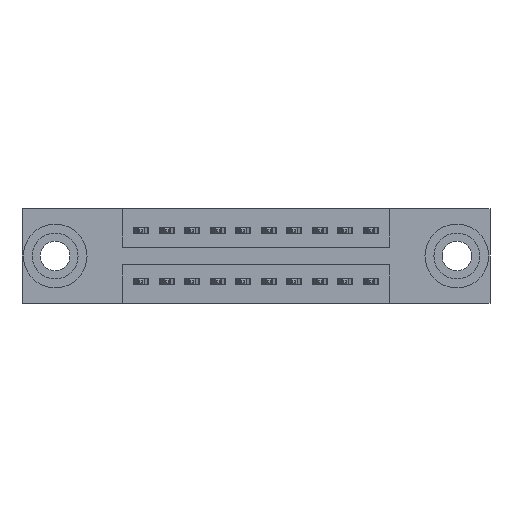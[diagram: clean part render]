
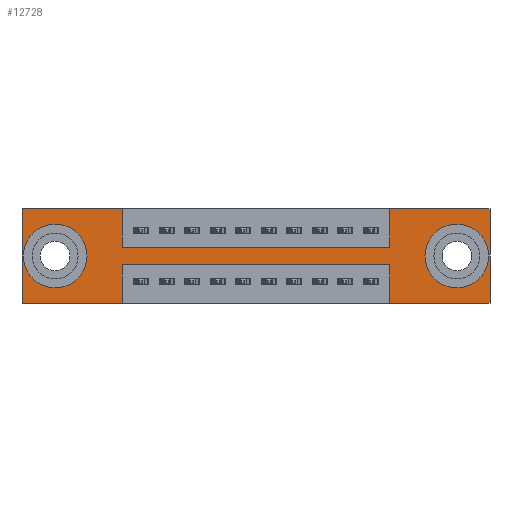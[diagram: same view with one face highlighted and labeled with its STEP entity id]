
A CAD part, front view. The second image highlights one B-rep face of the part: STEP entity #12728.
In plain terms, the highlighted planar face has unit normal (0, -1, 0).
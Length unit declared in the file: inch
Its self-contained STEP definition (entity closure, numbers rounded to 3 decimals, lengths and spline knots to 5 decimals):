
#14 = AXIS2_PLACEMENT_3D ( 'NONE', #4909, #11758, #6761 ) ;
#334 = CARTESIAN_POINT ( 'NONE',  ( 0.13, 0., -0.263 ) ) ;
#363 = VERTEX_POINT ( 'NONE', #11175 ) ;
#401 = FACE_BOUND ( 'NONE', #1657, .T. ) ;
#403 = VERTEX_POINT ( 'NONE', #590 ) ;
#487 = DIRECTION ( 'NONE',  ( 0., 0., -1. ) ) ;
#520 = CARTESIAN_POINT ( 'NONE',  ( 0., 0., -0.37 ) ) ;
#588 = ORIENTED_EDGE ( 'NONE', *, *, #11525, .F. ) ;
#590 = CARTESIAN_POINT ( 'NONE',  ( 1.4425, 0., -0.22 ) ) ;
#640 = CARTESIAN_POINT ( 'NONE',  ( 0., 0., 0. ) ) ;
#661 = DIRECTION ( 'NONE',  ( 1., 0., 0. ) ) ;
#730 = CARTESIAN_POINT ( 'NONE',  ( 1.705, 0., -0.263 ) ) ;
#820 = LINE ( 'NONE', #1407, #5165 ) ;
#821 = CARTESIAN_POINT ( 'NONE',  ( 1.4425, 0., 0. ) ) ;
#918 = VECTOR ( 'NONE', #2035, 39.37008 ) ;
#952 = EDGE_CURVE ( 'NONE', #6450, #5616, #7505, .T. ) ;
#1049 = CARTESIAN_POINT ( 'NONE',  ( 1.4425, 0., -0.15 ) ) ;
#1187 = VERTEX_POINT ( 'NONE', #2558 ) ;
#1219 = LINE ( 'NONE', #2517, #7746 ) ;
#1407 = CARTESIAN_POINT ( 'NONE',  ( 0.3925, 0., 0. ) ) ;
#1420 = VERTEX_POINT ( 'NONE', #9969 ) ;
#1519 = ORIENTED_EDGE ( 'NONE', *, *, #2421, .T. ) ;
#1657 = EDGE_LOOP ( 'NONE', ( #1519, #3399 ) ) ;
#1875 = LINE ( 'NONE', #9448, #12048 ) ;
#2007 = ORIENTED_EDGE ( 'NONE', *, *, #8410, .F. ) ;
#2035 = DIRECTION ( 'NONE',  ( 1., 0., 0. ) ) ;
#2104 = EDGE_CURVE ( 'NONE', #7133, #9747, #8995, .T. ) ;
#2215 = DIRECTION ( 'NONE',  ( 0., 0., -1. ) ) ;
#2421 = EDGE_CURVE ( 'NONE', #5616, #6450, #4376, .T. ) ;
#2428 = ORIENTED_EDGE ( 'NONE', *, *, #3195, .F. ) ;
#2517 = CARTESIAN_POINT ( 'NONE',  ( 1.4425, 0., 0. ) ) ;
#2558 = CARTESIAN_POINT ( 'NONE',  ( 0.3925, 0., -0.15 ) ) ;
#2655 = EDGE_CURVE ( 'NONE', #5471, #5787, #1875, .T. ) ;
#2875 = DIRECTION ( 'NONE',  ( 0., 1., 0. ) ) ;
#3140 = LINE ( 'NONE', #12783, #12194 ) ;
#3195 = EDGE_CURVE ( 'NONE', #12616, #7133, #1219, .T. ) ;
#3303 = AXIS2_PLACEMENT_3D ( 'NONE', #11957, #11881, #6075 ) ;
#3399 = ORIENTED_EDGE ( 'NONE', *, *, #952, .T. ) ;
#3496 = CIRCLE ( 'NONE', #6988, 0.078 ) ;
#3520 = LINE ( 'NONE', #3662, #4610 ) ;
#3662 = CARTESIAN_POINT ( 'NONE',  ( 1.4425, 0., -0.37 ) ) ;
#3936 = LINE ( 'NONE', #9445, #918 ) ;
#4036 = DIRECTION ( 'NONE',  ( -1., 0., 0. ) ) ;
#4045 = LINE ( 'NONE', #8840, #9701 ) ;
#4166 = EDGE_LOOP ( 'NONE', ( #6085, #7934, #2007, #10988, #8761, #10795, #2428, #588, #9913, #10186, #12549, #9404 ) ) ;
#4269 = PLANE ( 'NONE',  #6240 ) ;
#4342 = CARTESIAN_POINT ( 'NONE',  ( 1.705, 0., -0.107 ) ) ;
#4351 = DIRECTION ( 'NONE',  ( 0., 0., 1. ) ) ;
#4376 = CIRCLE ( 'NONE', #3303, 0.078 ) ;
#4523 = DIRECTION ( 'NONE',  ( -1., 0., 0. ) ) ;
#4610 = VECTOR ( 'NONE', #6633, 39.37008 ) ;
#4664 = DIRECTION ( 'NONE',  ( 0., 0., 1. ) ) ;
#4696 = VECTOR ( 'NONE', #12406, 39.37008 ) ;
#4839 = LINE ( 'NONE', #7964, #9729 ) ;
#4909 = CARTESIAN_POINT ( 'NONE',  ( 1.705, 0., -0.185 ) ) ;
#5046 = VERTEX_POINT ( 'NONE', #12230 ) ;
#5165 = VECTOR ( 'NONE', #9189, 39.37008 ) ;
#5357 = ORIENTED_EDGE ( 'NONE', *, *, #7483, .T. ) ;
#5389 = DIRECTION ( 'NONE',  ( 0., 1., 0. ) ) ;
#5471 = VERTEX_POINT ( 'NONE', #7657 ) ;
#5484 = VERTEX_POINT ( 'NONE', #9618 ) ;
#5616 = VERTEX_POINT ( 'NONE', #4342 ) ;
#5787 = VERTEX_POINT ( 'NONE', #6535 ) ;
#5894 = VECTOR ( 'NONE', #661, 39.37008 ) ;
#5907 = LINE ( 'NONE', #520, #12192 ) ;
#5917 = CARTESIAN_POINT ( 'NONE',  ( 1.835, 0., 0. ) ) ;
#6075 = DIRECTION ( 'NONE',  ( 0., 0., -1. ) ) ;
#6085 = ORIENTED_EDGE ( 'NONE', *, *, #11815, .F. ) ;
#6240 = AXIS2_PLACEMENT_3D ( 'NONE', #7324, #9336, #487 ) ;
#6242 = CARTESIAN_POINT ( 'NONE',  ( 1.835, 0., -0.37 ) ) ;
#6280 = CARTESIAN_POINT ( 'NONE',  ( 0.13, 0., -0.185 ) ) ;
#6333 = FACE_OUTER_BOUND ( 'NONE', #4166, .T. ) ;
#6377 = CARTESIAN_POINT ( 'NONE',  ( 1.835, 0., 0. ) ) ;
#6450 = VERTEX_POINT ( 'NONE', #730 ) ;
#6535 = CARTESIAN_POINT ( 'NONE',  ( 0., 0., -0.37 ) ) ;
#6633 = DIRECTION ( 'NONE',  ( 0., 0., 1. ) ) ;
#6761 = DIRECTION ( 'NONE',  ( 0., 0., -1. ) ) ;
#6924 = ORIENTED_EDGE ( 'NONE', *, *, #8268, .T. ) ;
#6988 = AXIS2_PLACEMENT_3D ( 'NONE', #6280, #5389, #4351 ) ;
#7120 = FACE_BOUND ( 'NONE', #7446, .T. ) ;
#7133 = VERTEX_POINT ( 'NONE', #821 ) ;
#7213 = CARTESIAN_POINT ( 'NONE',  ( 0.3925, 0., 0. ) ) ;
#7307 = DIRECTION ( 'NONE',  ( -1., 0., 0. ) ) ;
#7323 = DIRECTION ( 'NONE',  ( 0., 0., 1. ) ) ;
#7324 = CARTESIAN_POINT ( 'NONE',  ( 0., 0., -0.37 ) ) ;
#7445 = LINE ( 'NONE', #7785, #5894 ) ;
#7446 = EDGE_LOOP ( 'NONE', ( #6924, #5357 ) ) ;
#7483 = EDGE_CURVE ( 'NONE', #10103, #363, #3496, .T. ) ;
#7505 = CIRCLE ( 'NONE', #14, 0.078 ) ;
#7515 = CIRCLE ( 'NONE', #9828, 0.078 ) ;
#7530 = EDGE_CURVE ( 'NONE', #11587, #1187, #820, .T. ) ;
#7657 = CARTESIAN_POINT ( 'NONE',  ( 0.3925, 0., -0.37 ) ) ;
#7746 = VECTOR ( 'NONE', #7323, 39.37008 ) ;
#7785 = CARTESIAN_POINT ( 'NONE',  ( 0.3925, 0., -0.15 ) ) ;
#7934 = ORIENTED_EDGE ( 'NONE', *, *, #12562, .F. ) ;
#7964 = CARTESIAN_POINT ( 'NONE',  ( 0., 0., 0. ) ) ;
#8091 = EDGE_CURVE ( 'NONE', #5046, #11587, #3936, .T. ) ;
#8268 = EDGE_CURVE ( 'NONE', #363, #10103, #7515, .T. ) ;
#8410 = EDGE_CURVE ( 'NONE', #5484, #403, #3520, .T. ) ;
#8761 = ORIENTED_EDGE ( 'NONE', *, *, #11613, .F. ) ;
#8840 = CARTESIAN_POINT ( 'NONE',  ( 0.3925, 0., -0.22 ) ) ;
#8995 = LINE ( 'NONE', #640, #12218 ) ;
#9189 = DIRECTION ( 'NONE',  ( 0., 0., -1. ) ) ;
#9275 = LINE ( 'NONE', #6377, #4696 ) ;
#9336 = DIRECTION ( 'NONE',  ( 0., -1., 0. ) ) ;
#9340 = DIRECTION ( 'NONE',  ( 0., 0., 1. ) ) ;
#9404 = ORIENTED_EDGE ( 'NONE', *, *, #2655, .F. ) ;
#9445 = CARTESIAN_POINT ( 'NONE',  ( 0., 0., 0. ) ) ;
#9448 = CARTESIAN_POINT ( 'NONE',  ( 0., 0., -0.37 ) ) ;
#9560 = DIRECTION ( 'NONE',  ( 1., 0., 0. ) ) ;
#9618 = CARTESIAN_POINT ( 'NONE',  ( 1.4425, 0., -0.37 ) ) ;
#9701 = VECTOR ( 'NONE', #4036, 39.37008 ) ;
#9729 = VECTOR ( 'NONE', #9340, 39.37008 ) ;
#9747 = VERTEX_POINT ( 'NONE', #5917 ) ;
#9828 = AXIS2_PLACEMENT_3D ( 'NONE', #11638, #2875, #4664 ) ;
#9882 = VERTEX_POINT ( 'NONE', #6242 ) ;
#9913 = ORIENTED_EDGE ( 'NONE', *, *, #7530, .F. ) ;
#9969 = CARTESIAN_POINT ( 'NONE',  ( 0.3925, 0., -0.22 ) ) ;
#10103 = VERTEX_POINT ( 'NONE', #334 ) ;
#10186 = ORIENTED_EDGE ( 'NONE', *, *, #8091, .F. ) ;
#10795 = ORIENTED_EDGE ( 'NONE', *, *, #2104, .F. ) ;
#10988 = ORIENTED_EDGE ( 'NONE', *, *, #11168, .F. ) ;
#11168 = EDGE_CURVE ( 'NONE', #9882, #5484, #5907, .T. ) ;
#11175 = CARTESIAN_POINT ( 'NONE',  ( 0.13, 0., -0.107 ) ) ;
#11525 = EDGE_CURVE ( 'NONE', #1187, #12616, #7445, .T. ) ;
#11587 = VERTEX_POINT ( 'NONE', #7213 ) ;
#11595 = EDGE_CURVE ( 'NONE', #5787, #5046, #4839, .T. ) ;
#11613 = EDGE_CURVE ( 'NONE', #9747, #9882, #9275, .T. ) ;
#11638 = CARTESIAN_POINT ( 'NONE',  ( 0.13, 0., -0.185 ) ) ;
#11758 = DIRECTION ( 'NONE',  ( 0., 1., 0. ) ) ;
#11815 = EDGE_CURVE ( 'NONE', #1420, #5471, #3140, .T. ) ;
#11881 = DIRECTION ( 'NONE',  ( 0., 1., 0. ) ) ;
#11957 = CARTESIAN_POINT ( 'NONE',  ( 1.705, 0., -0.185 ) ) ;
#12048 = VECTOR ( 'NONE', #4523, 39.37008 ) ;
#12192 = VECTOR ( 'NONE', #7307, 39.37008 ) ;
#12194 = VECTOR ( 'NONE', #2215, 39.37008 ) ;
#12218 = VECTOR ( 'NONE', #9560, 39.37008 ) ;
#12230 = CARTESIAN_POINT ( 'NONE',  ( 0., 0., 0. ) ) ;
#12406 = DIRECTION ( 'NONE',  ( 0., 0., -1. ) ) ;
#12549 = ORIENTED_EDGE ( 'NONE', *, *, #11595, .F. ) ;
#12562 = EDGE_CURVE ( 'NONE', #403, #1420, #4045, .T. ) ;
#12616 = VERTEX_POINT ( 'NONE', #1049 ) ;
#12728 = ADVANCED_FACE ( 'NONE', ( #401, #7120, #6333 ), #4269, .T. ) ;
#12783 = CARTESIAN_POINT ( 'NONE',  ( 0.3925, 0., -0.37 ) ) ;
